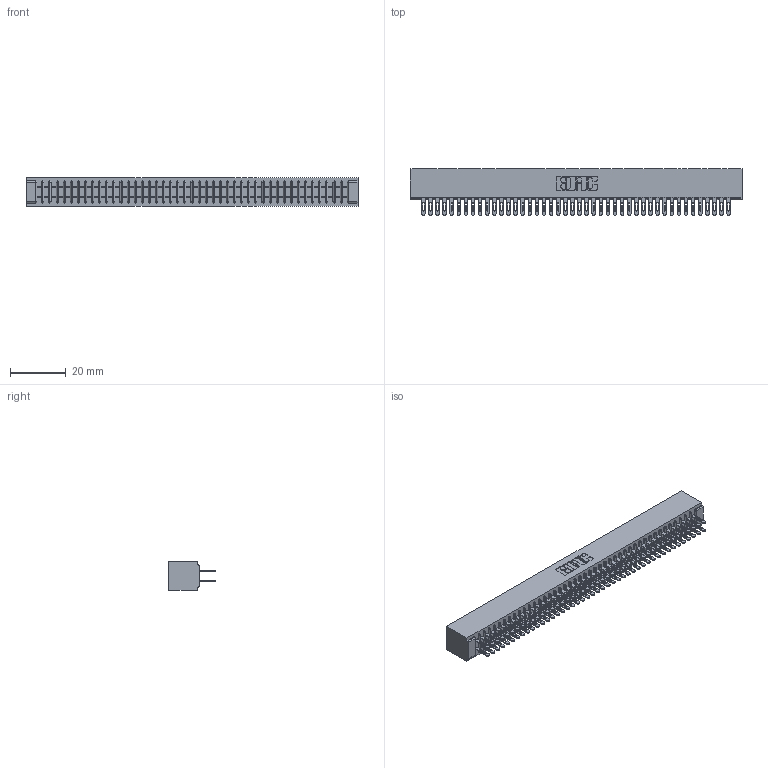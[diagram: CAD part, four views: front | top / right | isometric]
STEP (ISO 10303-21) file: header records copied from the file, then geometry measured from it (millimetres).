
FILE_DESCRIPTION (( 'STEP AP203' ), '1' );
FILE_NAME ('341-088-500-201.STEP', '2018-08-07T23:23:09', ( '' ), ( '' ), 'SwSTEP 2.0', 'SolidWorks 2016', '' );
FILE_SCHEMA (( 'CONFIG_CONTROL_DESIGN' ));
Length unit declared in the file: inch
Products named in the file (3): 341-088-500-201; 341 Part_No Mounting Lugs; 341-292-001_341-292-100
Assembly tree (89 placements, depth 2):
  341-088-500-201
    341 Part_No Mounting Lugs
    341-292-001_341-292-100  x88
Bounding box: 118.75 x 16.69 x 10.16 mm (x, y, z)
Volume: 9120 mm3; surface area: 17648.2 mm2
Topology: 89 solids, 89 shells, 5916 faces, 17144 edges, 11102 vertices
Faces by surface type: plane 3408, cylinder 2332, sphere 90, torus 86
Entity records: 52713 total; most frequent: CARTESIAN_POINT 8760, ORIENTED_EDGE 8704, DIRECTION 8502, EDGE_CURVE 4352, VECTOR 3518, LINE 3518, VERTEX_POINT 2750, AXIS2_PLACEMENT_3D 2492
